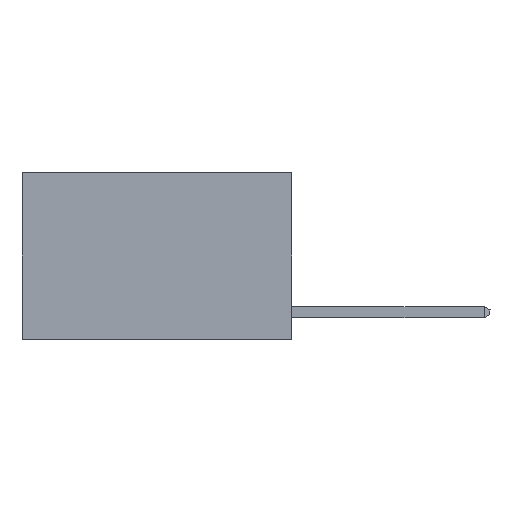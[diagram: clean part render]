
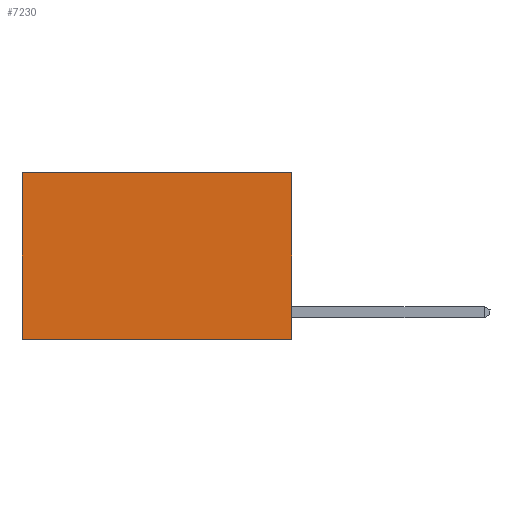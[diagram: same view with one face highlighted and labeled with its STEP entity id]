
A CAD part, left-side view. The second image highlights one B-rep face of the part: STEP entity #7230.
In plain terms, the highlighted planar face has unit normal (-1, 0, 0).
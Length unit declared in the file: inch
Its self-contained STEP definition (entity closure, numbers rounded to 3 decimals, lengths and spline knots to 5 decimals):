
#768 = LINE ( 'NONE', #12331, #5124 ) ;
#1029 = VERTEX_POINT ( 'NONE', #11885 ) ;
#1726 = DIRECTION ( 'NONE',  ( 0., 1., 0. ) ) ;
#2460 = VECTOR ( 'NONE', #1726, 39.37008 ) ;
#2798 = EDGE_CURVE ( 'NONE', #3163, #8536, #7169, .T. ) ;
#3163 = VERTEX_POINT ( 'NONE', #13611 ) ;
#3210 = ORIENTED_EDGE ( 'NONE', *, *, #9408, .T. ) ;
#3349 = LINE ( 'NONE', #11859, #18615 ) ;
#3716 = CARTESIAN_POINT ( 'NONE',  ( 0.2625, 0., 0. ) ) ;
#3939 = EDGE_CURVE ( 'NONE', #1029, #8536, #3349, .T. ) ;
#4017 = CARTESIAN_POINT ( 'NONE',  ( 0.2625, 0., -0.37 ) ) ;
#4903 = VECTOR ( 'NONE', #25702, 39.37008 ) ;
#5124 = VECTOR ( 'NONE', #15499, 39.37008 ) ;
#6332 = DIRECTION ( 'NONE',  ( 0., 0., -1. ) ) ;
#7169 = LINE ( 'NONE', #4017, #2460 ) ;
#7230 = ADVANCED_FACE ( 'NONE', ( #10049 ), #25385, .F. ) ;
#7750 = LINE ( 'NONE', #20301, #4903 ) ;
#8536 = VERTEX_POINT ( 'NONE', #17546 ) ;
#9408 = EDGE_CURVE ( 'NONE', #24386, #1029, #7750, .T. ) ;
#9513 = DIRECTION ( 'NONE',  ( 1., 0., 0. ) ) ;
#10049 = FACE_OUTER_BOUND ( 'NONE', #22458, .T. ) ;
#10735 = AXIS2_PLACEMENT_3D ( 'NONE', #15241, #9513, #23202 ) ;
#11859 = CARTESIAN_POINT ( 'NONE',  ( 0.2625, 0.6, 0. ) ) ;
#11885 = CARTESIAN_POINT ( 'NONE',  ( 0.2625, 0.6, 0. ) ) ;
#12331 = CARTESIAN_POINT ( 'NONE',  ( 0.2625, 0., 0. ) ) ;
#13611 = CARTESIAN_POINT ( 'NONE',  ( 0.2625, 0., -0.37 ) ) ;
#15241 = CARTESIAN_POINT ( 'NONE',  ( 0.2625, 0., 0. ) ) ;
#15499 = DIRECTION ( 'NONE',  ( 0., 0., -1. ) ) ;
#17546 = CARTESIAN_POINT ( 'NONE',  ( 0.2625, 0.6, -0.37 ) ) ;
#18615 = VECTOR ( 'NONE', #6332, 39.37008 ) ;
#18846 = ORIENTED_EDGE ( 'NONE', *, *, #3939, .T. ) ;
#20301 = CARTESIAN_POINT ( 'NONE',  ( 0.2625, 0., 0. ) ) ;
#22458 = EDGE_LOOP ( 'NONE', ( #18846, #22720, #24982, #3210 ) ) ;
#22720 = ORIENTED_EDGE ( 'NONE', *, *, #2798, .F. ) ;
#23202 = DIRECTION ( 'NONE',  ( 0., 0., -1. ) ) ;
#23640 = EDGE_CURVE ( 'NONE', #24386, #3163, #768, .T. ) ;
#24386 = VERTEX_POINT ( 'NONE', #3716 ) ;
#24982 = ORIENTED_EDGE ( 'NONE', *, *, #23640, .F. ) ;
#25385 = PLANE ( 'NONE',  #10735 ) ;
#25702 = DIRECTION ( 'NONE',  ( 0., 1., 0. ) ) ;
